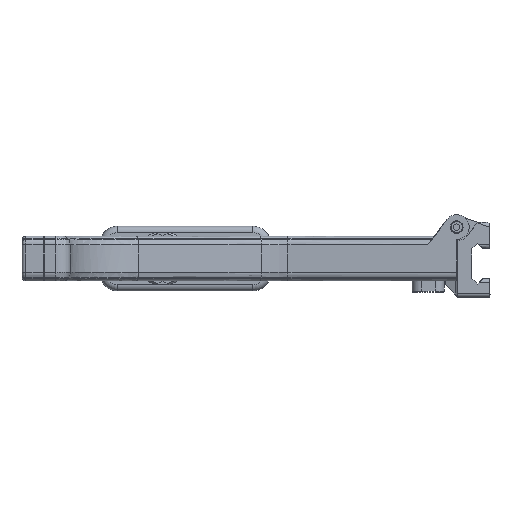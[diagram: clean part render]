
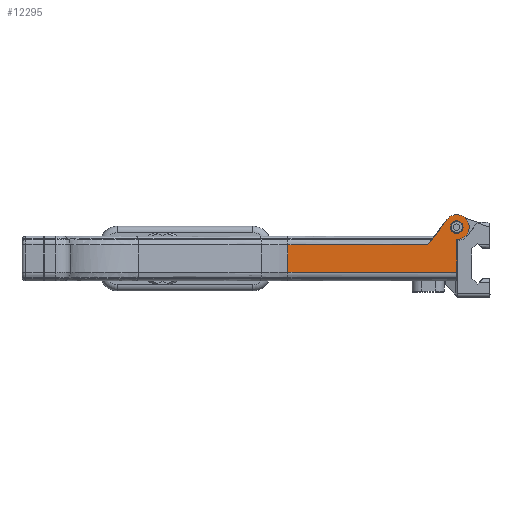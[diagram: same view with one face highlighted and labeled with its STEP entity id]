
A CAD part, front view. The second image highlights one B-rep face of the part: STEP entity #12295.
In plain terms, the highlighted planar face has unit normal (0, -1, 0).
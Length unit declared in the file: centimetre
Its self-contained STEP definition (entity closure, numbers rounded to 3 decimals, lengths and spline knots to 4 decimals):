
#448=FACE_BOUND($,#2470,.T.);
#760=CIRCLE($,#12813,0.35);
#895=CIRCLE($,#13181,0.69);
#1702=FACE_OUTER_BOUND($,#2469,.T.);
#2469=EDGE_LOOP($,(#9468,#9469,#9470,#9471,#9472,#9473));
#2470=EDGE_LOOP($,(#9474));
#3018=LINE($,#18198,#4028);
#3036=LINE($,#18336,#4046);
#3314=LINE($,#23794,#4324);
#3315=LINE($,#23796,#4325);
#3316=LINE($,#23797,#4326);
#4028=VECTOR($,#14187,1.7534);
#4046=VECTOR($,#14241,7.7816);
#4324=VECTOR($,#15297,1.5235);
#4325=VECTOR($,#15298,9.3876);
#4326=VECTOR($,#15299,1.8192);
#5080=VERTEX_POINT($,#18192);
#5081=VERTEX_POINT($,#18197);
#5104=VERTEX_POINT($,#18334);
#5106=VERTEX_POINT($,#18341);
#5399=VERTEX_POINT($,#23570);
#5409=VERTEX_POINT($,#23706);
#5410=VERTEX_POINT($,#23795);
#6281=EDGE_CURVE($,#5080,#5081,#3018,.T.);
#6316=EDGE_CURVE($,#5104,#5080,#3036,.T.);
#6318=EDGE_CURVE($,#5106,#5106,#760,.F.);
#6861=EDGE_CURVE($,#5399,#5081,#895,.T.);
#6888=EDGE_CURVE($,#5409,#5104,#3314,.T.);
#6889=EDGE_CURVE($,#5410,#5409,#3315,.T.);
#6890=EDGE_CURVE($,#5410,#5399,#3316,.F.);
#9468=ORIENTED_EDGE($,*,*,#6281,.F.);
#9469=ORIENTED_EDGE($,*,*,#6316,.F.);
#9470=ORIENTED_EDGE($,*,*,#6888,.F.);
#9471=ORIENTED_EDGE($,*,*,#6889,.F.);
#9472=ORIENTED_EDGE($,*,*,#6890,.T.);
#9473=ORIENTED_EDGE($,*,*,#6861,.T.);
#9474=ORIENTED_EDGE($,*,*,#6318,.T.);
#11778=PLANE($,#13198);
#12295=ADVANCED_FACE($,(#1702,#448),#11778,.T.);
#12813=AXIS2_PLACEMENT_3D($,#18342,#14248,#14249);
#13181=AXIS2_PLACEMENT_3D($,#23571,#15241,#15242);
#13198=AXIS2_PLACEMENT_3D($,#23793,#15295,#15296);
#14187=DIRECTION($,(0.602,0.,0.799));
#14241=DIRECTION($,(1.,0.,0.));
#14248=DIRECTION('center_axis',(0.,-1.,0.));
#14249=DIRECTION('ref_axis',(1.,0.,0.));
#15241=DIRECTION('center_axis',(0.,-1.,0.));
#15242=DIRECTION('ref_axis',(0.901,0.,0.433));
#15295=DIRECTION('center_axis',(0.,-1.,0.));
#15296=DIRECTION('ref_axis',(0.,0.,
-1.));
#15297=DIRECTION($,(0.,0.,1.));
#15298=DIRECTION($,(-1.,0.,0.));
#15299=DIRECTION($,(0.,0.,-1.));
#18192=CARTESIAN_POINT('',(-23.9508,-0.2943,1.1464));
#18197=CARTESIAN_POINT('',(-22.896,-0.2943,2.5472));
#18198=CARTESIAN_POINT($,(-23.5023,-0.2943,1.742));
#18334=CARTESIAN_POINT('',(-31.7324,-0.2943,1.1464));
#18336=CARTESIAN_POINT($,(-39.1636,-0.2943,1.1464));
#18341=CARTESIAN_POINT('',(-22.6948,-0.2943,2.1321));
#18342=CARTESIAN_POINT('Origin',(-22.3448,-0.2943,2.1321));
#23570=CARTESIAN_POINT('',(-22.3448,-0.2943,1.4421));
#23571=CARTESIAN_POINT('Origin',(-22.3448,-0.2943,2.1321));
#23706=CARTESIAN_POINT('',(-31.7324,-0.2943,-0.3771));
#23793=CARTESIAN_POINT('Origin',(-21.7548,-0.2943,-0.8603));
#23794=CARTESIAN_POINT($,(-31.7324,-0.2943,-1.1714));
#23795=CARTESIAN_POINT('',(-22.3448,-0.2943,-0.3771));
#23796=CARTESIAN_POINT($,(-36.9636,-0.2943,-0.3771));
#23797=CARTESIAN_POINT($,(-22.3448,-0.2943,0.3847));
